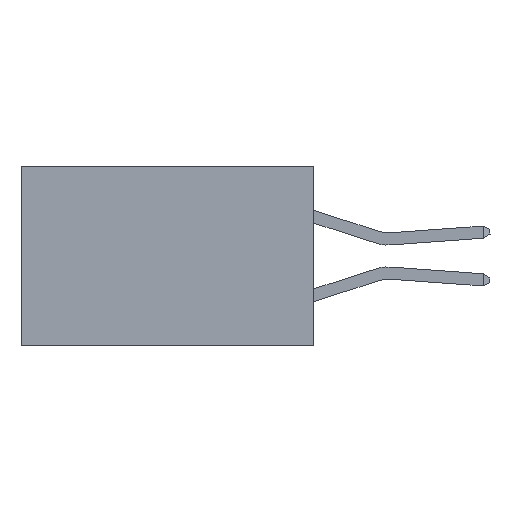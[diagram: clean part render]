
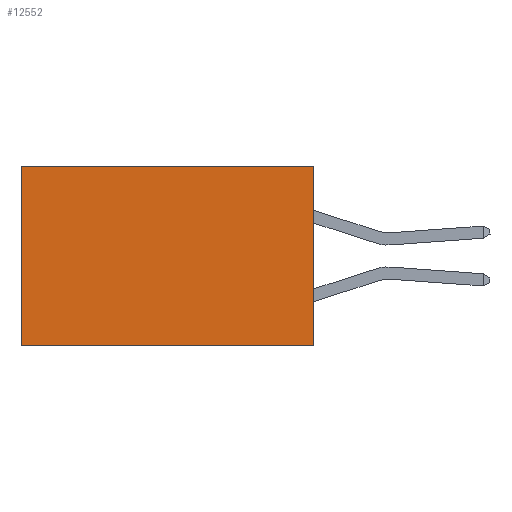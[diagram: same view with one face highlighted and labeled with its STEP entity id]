
A CAD part, left-side view. The second image highlights one B-rep face of the part: STEP entity #12552.
In plain terms, the highlighted planar face has unit normal (-1, 0, 0).
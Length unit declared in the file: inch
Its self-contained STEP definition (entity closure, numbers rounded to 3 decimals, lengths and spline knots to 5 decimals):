
#3346 = FACE_OUTER_BOUND ( 'NONE', #4754, .T. ) ;
#4066 = AXIS2_PLACEMENT_3D ( 'NONE', #20621, #32322, #5596 ) ;
#4754 = EDGE_LOOP ( 'NONE', ( #24852, #18881, #26234, #11413 ) ) ;
#5596 = DIRECTION ( 'NONE',  ( 0., 0., -1. ) ) ;
#6984 = CARTESIAN_POINT ( 'NONE',  ( 0.2875, 0., 0. ) ) ;
#7525 = DIRECTION ( 'NONE',  ( 0., 0., -1. ) ) ;
#8953 = DIRECTION ( 'NONE',  ( 0., 0., -1. ) ) ;
#9073 = LINE ( 'NONE', #6984, #37844 ) ;
#9342 = CARTESIAN_POINT ( 'NONE',  ( 0.2875, 0., -0.37 ) ) ;
#9409 = VECTOR ( 'NONE', #7525, 39.37008 ) ;
#10534 = CARTESIAN_POINT ( 'NONE',  ( 0.2875, 0., 0. ) ) ;
#11413 = ORIENTED_EDGE ( 'NONE', *, *, #32762, .T. ) ;
#12552 = ADVANCED_FACE ( 'NONE', ( #3346 ), #23641, .F. ) ;
#13035 = DIRECTION ( 'NONE',  ( 0., 1., 0. ) ) ;
#17735 = VERTEX_POINT ( 'NONE', #28750 ) ;
#18758 = VERTEX_POINT ( 'NONE', #27418 ) ;
#18881 = ORIENTED_EDGE ( 'NONE', *, *, #19390, .F. ) ;
#19390 = EDGE_CURVE ( 'NONE', #31980, #20364, #28769, .T. ) ;
#20364 = VERTEX_POINT ( 'NONE', #32045 ) ;
#20621 = CARTESIAN_POINT ( 'NONE',  ( 0.2875, 0., 0. ) ) ;
#20947 = VECTOR ( 'NONE', #27239, 39.37008 ) ;
#23641 = PLANE ( 'NONE',  #4066 ) ;
#24852 = ORIENTED_EDGE ( 'NONE', *, *, #32551, .T. ) ;
#26234 = ORIENTED_EDGE ( 'NONE', *, *, #28051, .F. ) ;
#26996 = CARTESIAN_POINT ( 'NONE',  ( 0.2875, 0.6, 0. ) ) ;
#27239 = DIRECTION ( 'NONE',  ( 0., 1., 0. ) ) ;
#27418 = CARTESIAN_POINT ( 'NONE',  ( 0.2875, 0.6, 0. ) ) ;
#28051 = EDGE_CURVE ( 'NONE', #17735, #31980, #33135, .T. ) ;
#28750 = CARTESIAN_POINT ( 'NONE',  ( 0.2875, 0., 0. ) ) ;
#28769 = LINE ( 'NONE', #9342, #20947 ) ;
#29076 = LINE ( 'NONE', #26996, #37797 ) ;
#31980 = VERTEX_POINT ( 'NONE', #32778 ) ;
#32045 = CARTESIAN_POINT ( 'NONE',  ( 0.2875, 0.6, -0.37 ) ) ;
#32322 = DIRECTION ( 'NONE',  ( 1., 0., 0. ) ) ;
#32551 = EDGE_CURVE ( 'NONE', #18758, #20364, #29076, .T. ) ;
#32762 = EDGE_CURVE ( 'NONE', #17735, #18758, #9073, .T. ) ;
#32778 = CARTESIAN_POINT ( 'NONE',  ( 0.2875, 0., -0.37 ) ) ;
#33135 = LINE ( 'NONE', #10534, #9409 ) ;
#37797 = VECTOR ( 'NONE', #8953, 39.37008 ) ;
#37844 = VECTOR ( 'NONE', #13035, 39.37008 ) ;
